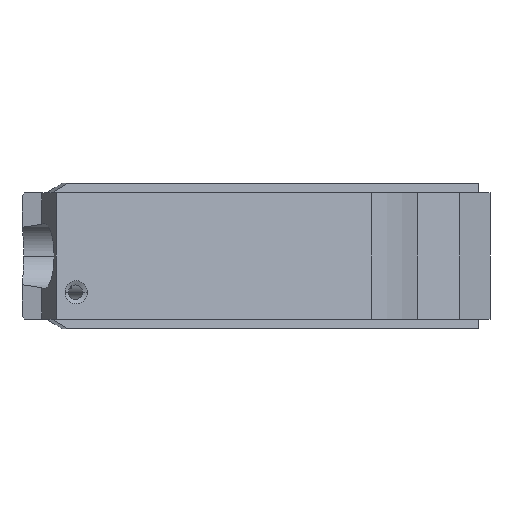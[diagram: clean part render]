
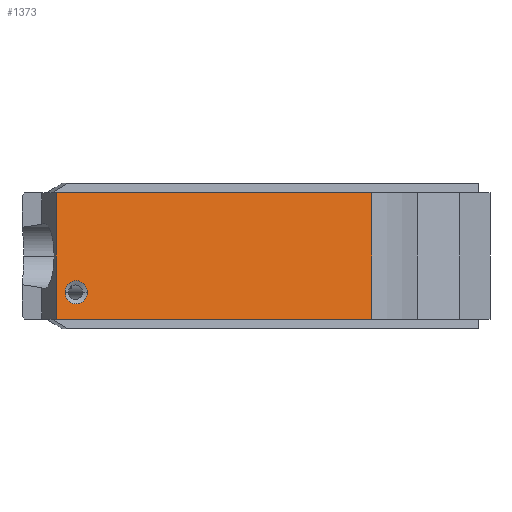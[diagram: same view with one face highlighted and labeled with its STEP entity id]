
A CAD part, left-side view. The second image highlights one B-rep face of the part: STEP entity #1373.
In plain terms, the highlighted planar face has unit normal (-0.954, -0.301, 0).
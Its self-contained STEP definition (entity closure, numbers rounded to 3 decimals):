
#24=DIRECTION('',(-0.301,0.954,0.));
#25=VECTOR('',#24,35.814);
#26=CARTESIAN_POINT('',(89.37,-83.115,6.833));
#27=LINE('',#26,#25);
#113=DIRECTION('',(0.301,-0.954,0.));
#114=VECTOR('',#113,35.814);
#115=CARTESIAN_POINT('',(78.6,-48.959,-6.833));
#116=LINE('',#115,#114);
#275=DIRECTION('',(0.,0.,-1.));
#276=VECTOR('',#275,13.665);
#277=CARTESIAN_POINT('',(78.6,-48.959,6.833));
#278=LINE('',#277,#276);
#548=CARTESIAN_POINT('',(79.272,-51.09,-3.937));
#549=DIRECTION('',(-0.954,-0.301,0.));
#550=DIRECTION('',(-0.301,0.954,0.));
#551=AXIS2_PLACEMENT_3D('',#548,#549,#550);
#553=CARTESIAN_POINT('',(79.272,-51.09,-3.937));
#554=DIRECTION('',(-0.954,-0.301,0.));
#555=DIRECTION('',(0.301,-0.954,0.));
#556=AXIS2_PLACEMENT_3D('',#553,#554,#555);
#562=DIRECTION('',(0.,0.,1.));
#563=VECTOR('',#562,13.665);
#564=CARTESIAN_POINT('',(89.37,-83.115,-6.833));
#565=LINE('',#564,#563);
#654=CARTESIAN_POINT('',(89.37,-83.115,6.833));
#655=VERTEX_POINT('',#654);
#656=CARTESIAN_POINT('',(78.6,-48.959,6.833));
#657=VERTEX_POINT('',#656);
#684=CARTESIAN_POINT('',(78.6,-48.959,-6.833));
#685=VERTEX_POINT('',#684);
#694=CARTESIAN_POINT('',(89.37,-83.115,-6.833));
#695=VERTEX_POINT('',#694);
#702=CARTESIAN_POINT('',(78.894,-49.891,-3.937));
#703=CARTESIAN_POINT('',(79.65,-52.289,-3.937));
#704=VERTEX_POINT('',#702);
#705=VERTEX_POINT('',#703);
#1357=CARTESIAN_POINT('',(83.985,-66.037,0.));
#1358=DIRECTION('',(0.954,0.301,0.));
#1359=DIRECTION('',(0.301,-0.954,0.));
#1360=AXIS2_PLACEMENT_3D('',#1357,#1358,#1359);
#1361=PLANE('',#1360);
#1363=ORIENTED_EDGE('',*,*,#1362,.F.);
#1364=ORIENTED_EDGE('',*,*,#863,.F.);
#1365=ORIENTED_EDGE('',*,*,#1157,.F.);
#1366=ORIENTED_EDGE('',*,*,#783,.F.);
#1367=EDGE_LOOP('',(#1363,#1364,#1365,#1366));
#1368=FACE_OUTER_BOUND('',#1367,.F.);
#1369=ORIENTED_EDGE('',*,*,#1337,.T.);
#1370=ORIENTED_EDGE('',*,*,#1350,.T.);
#1371=EDGE_LOOP('',(#1369,#1370));
#1372=FACE_BOUND('',#1371,.F.);
#1373=ADVANCED_FACE('',(#1368,#1372),#1361,.F.);
#552=CIRCLE('',#551,1.257);
#557=CIRCLE('',#556,1.257);
#783=EDGE_CURVE('',#655,#657,#27,.T.);
#863=EDGE_CURVE('',#685,#695,#116,.T.);
#1157=EDGE_CURVE('',#657,#685,#278,.T.);
#1337=EDGE_CURVE('',#704,#705,#552,.T.);
#1350=EDGE_CURVE('',#705,#704,#557,.T.);
#1362=EDGE_CURVE('',#695,#655,#565,.T.);
